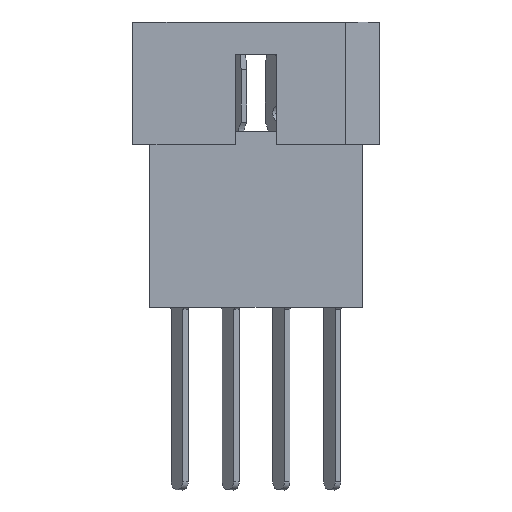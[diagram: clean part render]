
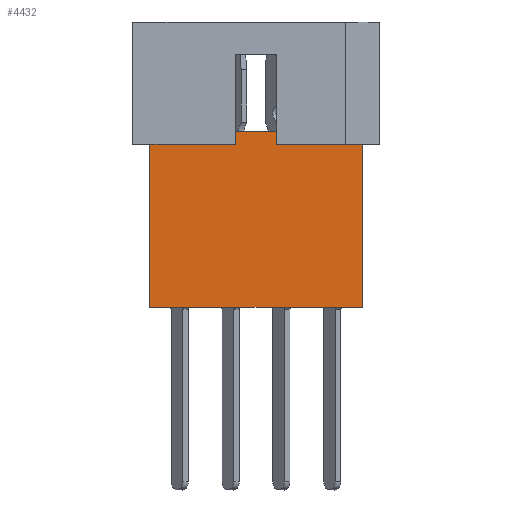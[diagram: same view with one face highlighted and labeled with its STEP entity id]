
A CAD part, top view. The second image highlights one B-rep face of the part: STEP entity #4432.
In plain terms, the highlighted planar face has unit normal (0, 0, 1).
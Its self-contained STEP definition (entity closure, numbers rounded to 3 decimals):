
#63 = LINE ( 'NONE', #2776, #2654 ) ;
#126 = CARTESIAN_POINT ( 'NONE',  ( 7.544, 0., 2.54 ) ) ;
#372 = DIRECTION ( 'NONE',  ( 0., -1., 0. ) ) ;
#574 = EDGE_CURVE ( 'NONE', #3640, #944, #658, .T. ) ;
#658 = LINE ( 'NONE', #703, #3623 ) ;
#703 = CARTESIAN_POINT ( 'NONE',  ( -2.324, 0., 2.54 ) ) ;
#766 = DIRECTION ( 'NONE',  ( 0., 1., 0. ) ) ;
#792 = CARTESIAN_POINT ( 'NONE',  ( -2.324, -12.7, 2.54 ) ) ;
#944 = VERTEX_POINT ( 'NONE', #7301 ) ;
#1151 = LINE ( 'NONE', #1325, #4115 ) ;
#1288 = ORIENTED_EDGE ( 'NONE', *, *, #6525, .F. ) ;
#1325 = CARTESIAN_POINT ( 'NONE',  ( -2.324, -12.7, 2.54 ) ) ;
#1348 = EDGE_CURVE ( 'NONE', #1464, #5477, #2004, .T. ) ;
#1388 = EDGE_CURVE ( 'NONE', #1534, #5477, #5045, .T. ) ;
#1464 = VERTEX_POINT ( 'NONE', #2301 ) ;
#1479 = FACE_OUTER_BOUND ( 'NONE', #1873, .T. ) ;
#1534 = VERTEX_POINT ( 'NONE', #126 ) ;
#1537 = DIRECTION ( 'NONE',  ( 0., 1., 0. ) ) ;
#1873 = EDGE_LOOP ( 'NONE', ( #2314, #6104, #4802, #4047, #3555, #7339, #1288, #2578 ) ) ;
#1913 = DIRECTION ( 'NONE',  ( 1., 0., 0. ) ) ;
#2004 = LINE ( 'NONE', #6154, #2626 ) ;
#2257 = LINE ( 'NONE', #5313, #4223 ) ;
#2301 = CARTESIAN_POINT ( 'NONE',  ( 14.211, -12.7, 2.54 ) ) ;
#2314 = ORIENTED_EDGE ( 'NONE', *, *, #574, .F. ) ;
#2417 = CARTESIAN_POINT ( 'NONE',  ( -2.324, -12.7, 2.54 ) ) ;
#2437 = DIRECTION ( 'NONE',  ( 1., 0., 0. ) ) ;
#2566 = EDGE_CURVE ( 'NONE', #4657, #944, #5122, .T. ) ;
#2578 = ORIENTED_EDGE ( 'NONE', *, *, #2566, .T. ) ;
#2626 = VECTOR ( 'NONE', #1537, 1000. ) ;
#2654 = VECTOR ( 'NONE', #3968, 1000. ) ;
#2731 = CARTESIAN_POINT ( 'NONE',  ( 7.544, 1.016, 2.54 ) ) ;
#2776 = CARTESIAN_POINT ( 'NONE',  ( 0., 1.016, 2.54 ) ) ;
#2784 = EDGE_CURVE ( 'NONE', #1534, #4829, #2257, .T. ) ;
#3047 = DIRECTION ( 'NONE',  ( 0., 0., 1. ) ) ;
#3524 = EDGE_CURVE ( 'NONE', #3724, #1464, #1151, .T. ) ;
#3555 = ORIENTED_EDGE ( 'NONE', *, *, #1388, .F. ) ;
#3623 = VECTOR ( 'NONE', #4447, 1000. ) ;
#3640 = VERTEX_POINT ( 'NONE', #4000 ) ;
#3724 = VERTEX_POINT ( 'NONE', #2417 ) ;
#3898 = CARTESIAN_POINT ( 'NONE',  ( -2.324, 0., 2.54 ) ) ;
#3968 = DIRECTION ( 'NONE',  ( 1., 0., 0. ) ) ;
#4000 = CARTESIAN_POINT ( 'NONE',  ( -2.324, 0., 2.54 ) ) ;
#4047 = ORIENTED_EDGE ( 'NONE', *, *, #1348, .T. ) ;
#4115 = VECTOR ( 'NONE', #1913, 1000. ) ;
#4223 = VECTOR ( 'NONE', #766, 1000. ) ;
#4342 = CARTESIAN_POINT ( 'NONE',  ( 4.343, 6.985, 2.54 ) ) ;
#4432 = ADVANCED_FACE ( 'NONE', ( #1479 ), #6498, .T. ) ;
#4447 = DIRECTION ( 'NONE',  ( 1., 0., 0. ) ) ;
#4498 = CARTESIAN_POINT ( 'NONE',  ( -2.324, -12.7, 2.54 ) ) ;
#4657 = VERTEX_POINT ( 'NONE', #5404 ) ;
#4802 = ORIENTED_EDGE ( 'NONE', *, *, #3524, .T. ) ;
#4829 = VERTEX_POINT ( 'NONE', #2731 ) ;
#4902 = EDGE_CURVE ( 'NONE', #3724, #3640, #6699, .T. ) ;
#4947 = AXIS2_PLACEMENT_3D ( 'NONE', #792, #3047, #2437 ) ;
#5019 = DIRECTION ( 'NONE',  ( 0., 1., 0. ) ) ;
#5045 = LINE ( 'NONE', #3898, #5864 ) ;
#5122 = LINE ( 'NONE', #4342, #7196 ) ;
#5313 = CARTESIAN_POINT ( 'NONE',  ( 7.544, 6.985, 2.54 ) ) ;
#5404 = CARTESIAN_POINT ( 'NONE',  ( 4.343, 1.016, 2.54 ) ) ;
#5428 = CARTESIAN_POINT ( 'NONE',  ( 14.211, 0., 2.54 ) ) ;
#5448 = VECTOR ( 'NONE', #5019, 1000. ) ;
#5477 = VERTEX_POINT ( 'NONE', #5428 ) ;
#5864 = VECTOR ( 'NONE', #6688, 1000. ) ;
#6104 = ORIENTED_EDGE ( 'NONE', *, *, #4902, .F. ) ;
#6154 = CARTESIAN_POINT ( 'NONE',  ( 14.211, -12.7, 2.54 ) ) ;
#6498 = PLANE ( 'NONE',  #4947 ) ;
#6525 = EDGE_CURVE ( 'NONE', #4657, #4829, #63, .T. ) ;
#6688 = DIRECTION ( 'NONE',  ( 1., 0., 0. ) ) ;
#6699 = LINE ( 'NONE', #4498, #5448 ) ;
#7196 = VECTOR ( 'NONE', #372, 1000. ) ;
#7301 = CARTESIAN_POINT ( 'NONE',  ( 4.343, 0., 2.54 ) ) ;
#7339 = ORIENTED_EDGE ( 'NONE', *, *, #2784, .T. ) ;
